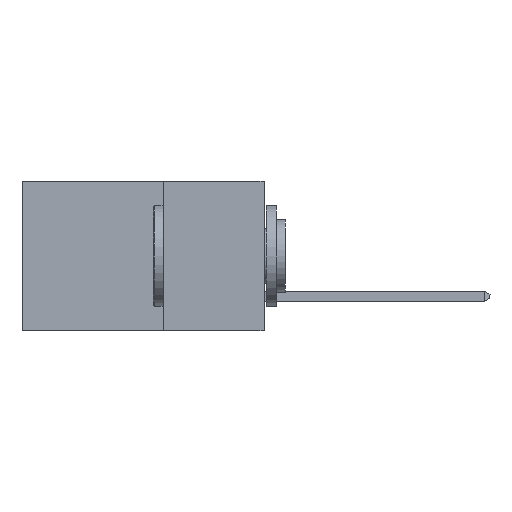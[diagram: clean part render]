
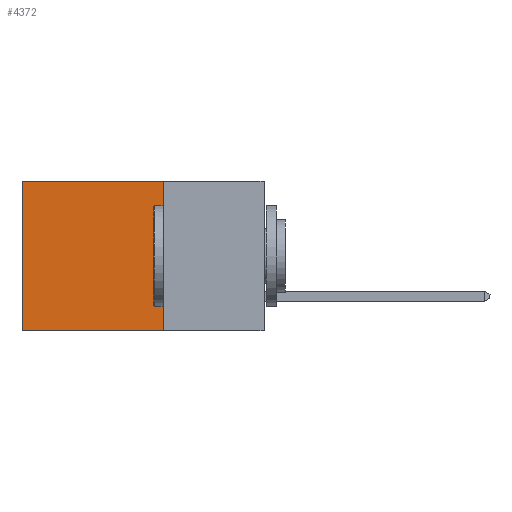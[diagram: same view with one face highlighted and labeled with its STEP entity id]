
A CAD part, left-side view. The second image highlights one B-rep face of the part: STEP entity #4372.
In plain terms, the highlighted planar face has unit normal (-1, 0, 0).
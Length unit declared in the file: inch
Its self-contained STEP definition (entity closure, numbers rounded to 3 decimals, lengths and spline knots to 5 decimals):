
#395 = EDGE_CURVE ( 'NONE', #10343, #3463, #5286, .T. ) ;
#407 = DIRECTION ( 'NONE',  ( 0., 0., -1. ) ) ;
#566 = ORIENTED_EDGE ( 'NONE', *, *, #3444, .F. ) ;
#1109 = ORIENTED_EDGE ( 'NONE', *, *, #395, .T. ) ;
#1694 = CARTESIAN_POINT ( 'NONE',  ( 0.2615, 0.25, -0.37 ) ) ;
#2021 = DIRECTION ( 'NONE',  ( 1., 0., 0. ) ) ;
#2052 = VECTOR ( 'NONE', #8508, 39.37008 ) ;
#2585 = ORIENTED_EDGE ( 'NONE', *, *, #8975, .F. ) ;
#2660 = CARTESIAN_POINT ( 'NONE',  ( 0.2615, 0.6, -0.37 ) ) ;
#3024 = DIRECTION ( 'NONE',  ( 0., 0., -1. ) ) ;
#3305 = VERTEX_POINT ( 'NONE', #2660 ) ;
#3441 = CARTESIAN_POINT ( 'NONE',  ( 0.2615, 0.25, -0.37 ) ) ;
#3444 = EDGE_CURVE ( 'NONE', #10343, #8526, #9895, .T. ) ;
#3463 = VERTEX_POINT ( 'NONE', #8229 ) ;
#3505 = FACE_OUTER_BOUND ( 'NONE', #9025, .T. ) ;
#4153 = ORIENTED_EDGE ( 'NONE', *, *, #7387, .T. ) ;
#4372 = ADVANCED_FACE ( 'NONE', ( #3505 ), #6696, .F. ) ;
#4381 = CARTESIAN_POINT ( 'NONE',  ( 0.2615, 0.25, 0. ) ) ;
#4392 = CARTESIAN_POINT ( 'NONE',  ( 0.2615, 0.25, 0. ) ) ;
#4613 = CARTESIAN_POINT ( 'NONE',  ( 0.2615, 0.25, -0.37 ) ) ;
#4699 = VECTOR ( 'NONE', #3024, 39.37008 ) ;
#4906 = DIRECTION ( 'NONE',  ( 0., 1., 0. ) ) ;
#5286 = LINE ( 'NONE', #4392, #2052 ) ;
#5544 = LINE ( 'NONE', #8737, #4699 ) ;
#6633 = DIRECTION ( 'NONE',  ( 0., 0., -1. ) ) ;
#6696 = PLANE ( 'NONE',  #7549 ) ;
#7387 = EDGE_CURVE ( 'NONE', #3463, #3305, #5544, .T. ) ;
#7523 = LINE ( 'NONE', #1694, #10067 ) ;
#7549 = AXIS2_PLACEMENT_3D ( 'NONE', #7599, #2021, #407 ) ;
#7599 = CARTESIAN_POINT ( 'NONE',  ( 0.2615, 0.25, -0.37 ) ) ;
#7865 = VECTOR ( 'NONE', #6633, 39.37008 ) ;
#8229 = CARTESIAN_POINT ( 'NONE',  ( 0.2615, 0.6, 0. ) ) ;
#8508 = DIRECTION ( 'NONE',  ( 0., 1., 0. ) ) ;
#8526 = VERTEX_POINT ( 'NONE', #4613 ) ;
#8737 = CARTESIAN_POINT ( 'NONE',  ( 0.2615, 0.6, -0.37 ) ) ;
#8975 = EDGE_CURVE ( 'NONE', #8526, #3305, #7523, .T. ) ;
#9025 = EDGE_LOOP ( 'NONE', ( #4153, #2585, #566, #1109 ) ) ;
#9895 = LINE ( 'NONE', #3441, #7865 ) ;
#10067 = VECTOR ( 'NONE', #4906, 39.37008 ) ;
#10343 = VERTEX_POINT ( 'NONE', #4381 ) ;
